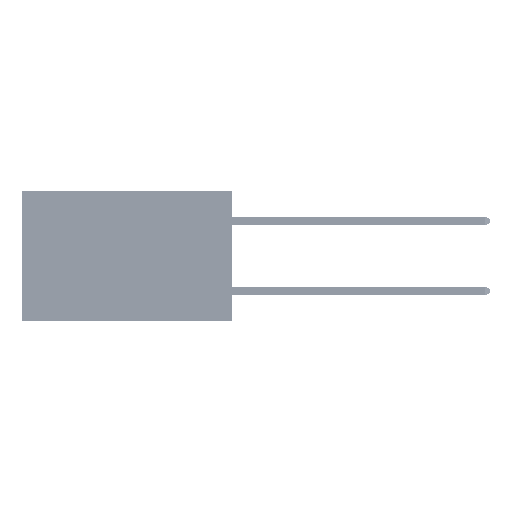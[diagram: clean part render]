
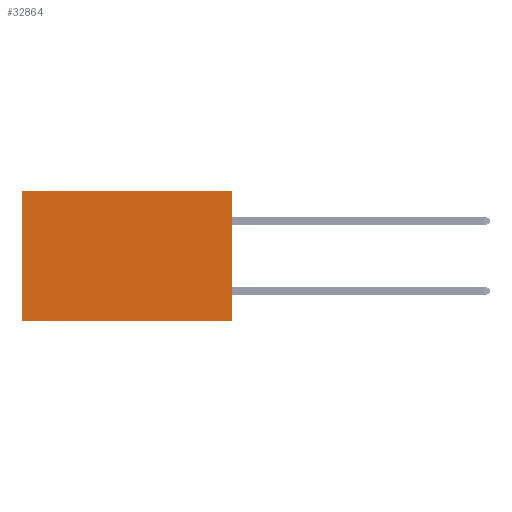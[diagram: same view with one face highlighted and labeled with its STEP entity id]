
A CAD part, left-side view. The second image highlights one B-rep face of the part: STEP entity #32864.
In plain terms, the highlighted planar face has unit normal (-1, 0, 0).
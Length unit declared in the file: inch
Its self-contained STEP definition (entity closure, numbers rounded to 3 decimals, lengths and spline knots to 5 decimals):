
#1443 = DIRECTION ( 'NONE',  ( 1., 0., 0. ) ) ;
#1775 = CARTESIAN_POINT ( 'NONE',  ( 0.2875, 0., 0. ) ) ;
#1843 = VERTEX_POINT ( 'NONE', #19774 ) ;
#3434 = DIRECTION ( 'NONE',  ( 0., 0., -1. ) ) ;
#4195 = LINE ( 'NONE', #15260, #44322 ) ;
#6170 = DIRECTION ( 'NONE',  ( 0., 0., -1. ) ) ;
#6315 = CARTESIAN_POINT ( 'NONE',  ( 0.2875, 0., 0. ) ) ;
#7624 = AXIS2_PLACEMENT_3D ( 'NONE', #1775, #1443, #17035 ) ;
#8182 = LINE ( 'NONE', #44996, #21521 ) ;
#8878 = EDGE_CURVE ( 'NONE', #33708, #1843, #8182, .T. ) ;
#9254 = EDGE_CURVE ( 'NONE', #15302, #26301, #29979, .T. ) ;
#9344 = VECTOR ( 'NONE', #22081, 39.37008 ) ;
#9736 = CARTESIAN_POINT ( 'NONE',  ( 0.2875, 0.6, 0. ) ) ;
#13130 = ORIENTED_EDGE ( 'NONE', *, *, #30619, .T. ) ;
#15260 = CARTESIAN_POINT ( 'NONE',  ( 0.2875, 0., 0. ) ) ;
#15302 = VERTEX_POINT ( 'NONE', #38394 ) ;
#16827 = EDGE_LOOP ( 'NONE', ( #13130, #23280, #28967, #49013 ) ) ;
#17035 = DIRECTION ( 'NONE',  ( 0., 0., -1. ) ) ;
#19774 = CARTESIAN_POINT ( 'NONE',  ( 0.2875, 0.6, -0.37 ) ) ;
#20312 = VECTOR ( 'NONE', #6170, 39.37008 ) ;
#21521 = VECTOR ( 'NONE', #25630, 39.37008 ) ;
#22034 = CARTESIAN_POINT ( 'NONE',  ( 0.2875, 0., -0.37 ) ) ;
#22081 = DIRECTION ( 'NONE',  ( 0., 1., 0. ) ) ;
#23280 = ORIENTED_EDGE ( 'NONE', *, *, #8878, .F. ) ;
#24692 = PLANE ( 'NONE',  #7624 ) ;
#25630 = DIRECTION ( 'NONE',  ( 0., 1., 0. ) ) ;
#26301 = VERTEX_POINT ( 'NONE', #36690 ) ;
#28967 = ORIENTED_EDGE ( 'NONE', *, *, #33179, .F. ) ;
#29979 = LINE ( 'NONE', #6315, #9344 ) ;
#30619 = EDGE_CURVE ( 'NONE', #26301, #1843, #36093, .T. ) ;
#32864 = ADVANCED_FACE ( 'NONE', ( #34016 ), #24692, .F. ) ;
#33179 = EDGE_CURVE ( 'NONE', #15302, #33708, #4195, .T. ) ;
#33708 = VERTEX_POINT ( 'NONE', #22034 ) ;
#34016 = FACE_OUTER_BOUND ( 'NONE', #16827, .T. ) ;
#36093 = LINE ( 'NONE', #9736, #20312 ) ;
#36690 = CARTESIAN_POINT ( 'NONE',  ( 0.2875, 0.6, 0. ) ) ;
#38394 = CARTESIAN_POINT ( 'NONE',  ( 0.2875, 0., 0. ) ) ;
#44322 = VECTOR ( 'NONE', #3434, 39.37008 ) ;
#44996 = CARTESIAN_POINT ( 'NONE',  ( 0.2875, 0., -0.37 ) ) ;
#49013 = ORIENTED_EDGE ( 'NONE', *, *, #9254, .T. ) ;
